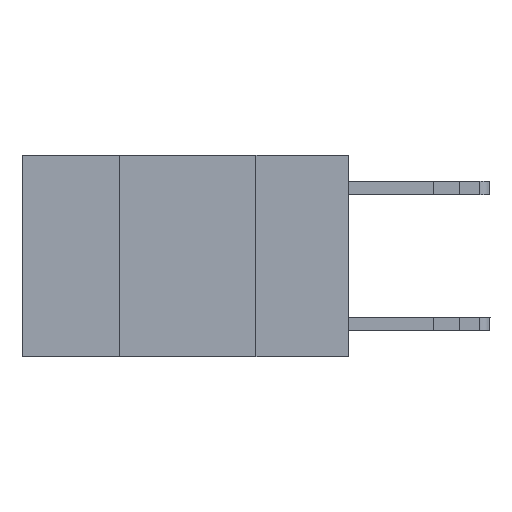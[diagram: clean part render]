
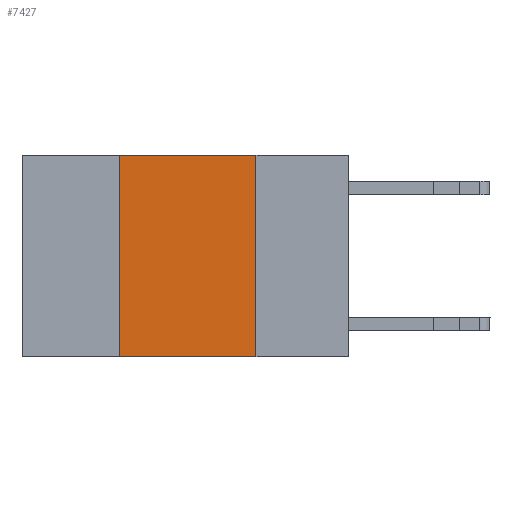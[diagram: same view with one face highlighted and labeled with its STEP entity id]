
A CAD part, left-side view. The second image highlights one B-rep face of the part: STEP entity #7427.
In plain terms, the highlighted planar face has unit normal (-1, 0, 0).
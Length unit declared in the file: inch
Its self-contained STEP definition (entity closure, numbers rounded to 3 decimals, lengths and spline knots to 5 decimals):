
#313 = LINE ( 'NONE', #18638, #578 ) ;
#578 = VECTOR ( 'NONE', #18678, 39.37008 ) ;
#1033 = ORIENTED_EDGE ( 'NONE', *, *, #2275, .T. ) ;
#2275 = EDGE_CURVE ( 'NONE', #16430, #4174, #313, .T. ) ;
#3598 = EDGE_CURVE ( 'NONE', #11942, #11975, #11768, .T. ) ;
#4070 = EDGE_LOOP ( 'NONE', ( #20721, #20262, #16985, #1033 ) ) ;
#4174 = VERTEX_POINT ( 'NONE', #12317 ) ;
#7427 = ADVANCED_FACE ( 'NONE', ( #17954 ), #19135, .F. ) ;
#8239 = VECTOR ( 'NONE', #16598, 39.37008 ) ;
#8480 = CARTESIAN_POINT ( 'NONE',  ( 0., 0.42, 0. ) ) ;
#8548 = DIRECTION ( 'NONE',  ( 0., 0., 1. ) ) ;
#8620 = LINE ( 'NONE', #18102, #8239 ) ;
#11694 = VECTOR ( 'NONE', #21060, 39.37008 ) ;
#11768 = LINE ( 'NONE', #21084, #11694 ) ;
#11942 = VERTEX_POINT ( 'NONE', #21276 ) ;
#11975 = VERTEX_POINT ( 'NONE', #20758 ) ;
#12317 = CARTESIAN_POINT ( 'NONE',  ( 0., 0.17, -0.37 ) ) ;
#16430 = VERTEX_POINT ( 'NONE', #18607 ) ;
#16598 = DIRECTION ( 'NONE',  ( 0., 0., -1. ) ) ;
#16985 = ORIENTED_EDGE ( 'NONE', *, *, #19239, .F. ) ;
#17954 = FACE_OUTER_BOUND ( 'NONE', #4070, .T. ) ;
#18102 = CARTESIAN_POINT ( 'NONE',  ( 0., 0.17, 0. ) ) ;
#18607 = CARTESIAN_POINT ( 'NONE',  ( 0., 0.42, -0.37 ) ) ;
#18625 = DIRECTION ( 'NONE',  ( 0., 0., -1. ) ) ;
#18638 = CARTESIAN_POINT ( 'NONE',  ( 0., 0.6, -0.37 ) ) ;
#18678 = DIRECTION ( 'NONE',  ( 0., -1., 0. ) ) ;
#18717 = DIRECTION ( 'NONE',  ( 1., 0., 0. ) ) ;
#19117 = CARTESIAN_POINT ( 'NONE',  ( 0., 0.6, 0. ) ) ;
#19135 = PLANE ( 'NONE',  #20362 ) ;
#19239 = EDGE_CURVE ( 'NONE', #16430, #11942, #19480, .T. ) ;
#19262 = VECTOR ( 'NONE', #8548, 39.37008 ) ;
#19480 = LINE ( 'NONE', #8480, #19262 ) ;
#20210 = EDGE_CURVE ( 'NONE', #11975, #4174, #8620, .T. ) ;
#20262 = ORIENTED_EDGE ( 'NONE', *, *, #3598, .F. ) ;
#20362 = AXIS2_PLACEMENT_3D ( 'NONE', #19117, #18717, #18625 ) ;
#20721 = ORIENTED_EDGE ( 'NONE', *, *, #20210, .F. ) ;
#20758 = CARTESIAN_POINT ( 'NONE',  ( 0., 0.17, 0. ) ) ;
#21060 = DIRECTION ( 'NONE',  ( 0., -1., 0. ) ) ;
#21084 = CARTESIAN_POINT ( 'NONE',  ( 0., 0.6, 0. ) ) ;
#21276 = CARTESIAN_POINT ( 'NONE',  ( 0., 0.42, 0. ) ) ;
